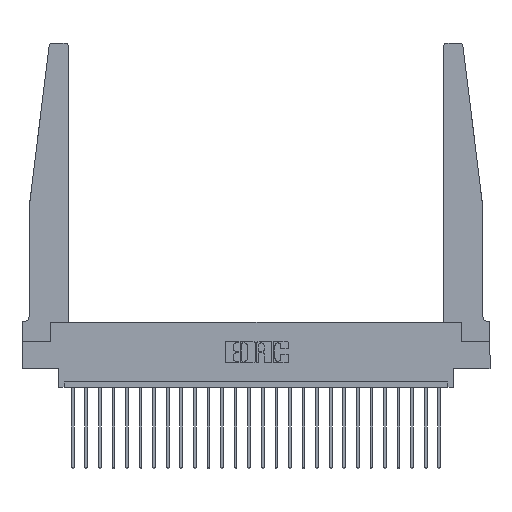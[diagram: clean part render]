
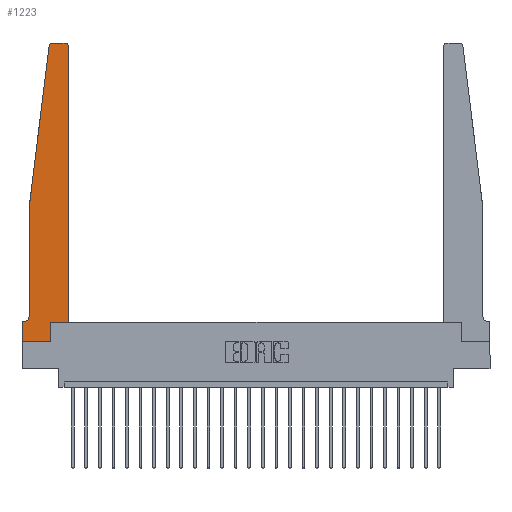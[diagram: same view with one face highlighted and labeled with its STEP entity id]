
A CAD part, top view. The second image highlights one B-rep face of the part: STEP entity #1223.
In plain terms, the highlighted planar face has unit normal (0, 0, 1).
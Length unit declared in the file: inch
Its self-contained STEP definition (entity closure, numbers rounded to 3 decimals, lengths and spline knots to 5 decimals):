
#128 = CARTESIAN_POINT ( 'NONE',  ( 0.425, 0.18, 0.37 ) ) ;
#375 = CIRCLE ( 'NONE', #13480, 0.05 ) ;
#581 = VERTEX_POINT ( 'NONE', #2257 ) ;
#605 = VERTEX_POINT ( 'NONE', #23213 ) ;
#639 = EDGE_CURVE ( 'NONE', #3316, #7666, #14233, .T. ) ;
#1006 = ORIENTED_EDGE ( 'NONE', *, *, #639, .T. ) ;
#1223 = ADVANCED_FACE ( 'NONE', ( #2860 ), #12051, .T. ) ;
#1259 = CARTESIAN_POINT ( 'NONE',  ( 0., 0., 0.37 ) ) ;
#1307 = VERTEX_POINT ( 'NONE', #23726 ) ;
#1462 = ORIENTED_EDGE ( 'NONE', *, *, #21147, .T. ) ;
#1631 = VERTEX_POINT ( 'NONE', #128 ) ;
#1940 = DIRECTION ( 'NONE',  ( 0., 1., 0. ) ) ;
#2257 = CARTESIAN_POINT ( 'NONE',  ( 0.065, 0.2375, 0.37 ) ) ;
#2538 = VERTEX_POINT ( 'NONE', #12047 ) ;
#2718 = VERTEX_POINT ( 'NONE', #4302 ) ;
#2796 = VERTEX_POINT ( 'NONE', #19030 ) ;
#2860 = FACE_OUTER_BOUND ( 'NONE', #19602, .T. ) ;
#3221 = VECTOR ( 'NONE', #15446, 39.37008 ) ;
#3316 = VERTEX_POINT ( 'NONE', #3672 ) ;
#3336 = CARTESIAN_POINT ( 'NONE',  ( 0.065, 0.1875, 0.37 ) ) ;
#3425 = DIRECTION ( 'NONE',  ( -1., 0., 0. ) ) ;
#3672 = CARTESIAN_POINT ( 'NONE',  ( 0., 0.1875, 0.37 ) ) ;
#4198 = VERTEX_POINT ( 'NONE', #4567 ) ;
#4255 = EDGE_CURVE ( 'NONE', #4198, #1307, #8488, .T. ) ;
#4270 = DIRECTION ( 'NONE',  ( 0., 0., 1. ) ) ;
#4302 = CARTESIAN_POINT ( 'NONE',  ( 0.2605, 0., 0.37 ) ) ;
#4433 = LINE ( 'NONE', #18751, #10799 ) ;
#4500 = AXIS2_PLACEMENT_3D ( 'NONE', #13820, #4270, #19492 ) ;
#4567 = CARTESIAN_POINT ( 'NONE',  ( 0.27653, 2.75, 0.37 ) ) ;
#4936 = CARTESIAN_POINT ( 'NONE',  ( 0.015, 0.2375, 0.37 ) ) ;
#5046 = CARTESIAN_POINT ( 'NONE',  ( 0.27653, 2.72, 0.37 ) ) ;
#5383 = EDGE_CURVE ( 'NONE', #2718, #605, #4433, .T. ) ;
#5413 = LINE ( 'NONE', #14546, #8006 ) ;
#5781 = DIRECTION ( 'NONE',  ( 0., 1., 0. ) ) ;
#5889 = DIRECTION ( 'NONE',  ( -0.122, -0.992, 0. ) ) ;
#6013 = CARTESIAN_POINT ( 'NONE',  ( 0.425, 0.18, 0.37 ) ) ;
#6110 = EDGE_CURVE ( 'NONE', #581, #23086, #375, .T. ) ;
#6342 = EDGE_CURVE ( 'NONE', #605, #1631, #12838, .T. ) ;
#6957 = ORIENTED_EDGE ( 'NONE', *, *, #10444, .T. ) ;
#7152 = VECTOR ( 'NONE', #21463, 39.37008 ) ;
#7315 = ORIENTED_EDGE ( 'NONE', *, *, #20209, .T. ) ;
#7651 = LINE ( 'NONE', #3336, #17643 ) ;
#7666 = VERTEX_POINT ( 'NONE', #1259 ) ;
#7957 = AXIS2_PLACEMENT_3D ( 'NONE', #15280, #22581, #18867 ) ;
#8006 = VECTOR ( 'NONE', #3425, 39.37008 ) ;
#8488 = CIRCLE ( 'NONE', #20848, 0.03 ) ;
#9393 = ORIENTED_EDGE ( 'NONE', *, *, #6110, .T. ) ;
#9825 = EDGE_CURVE ( 'NONE', #1631, #2796, #13906, .T. ) ;
#10371 = DIRECTION ( 'NONE',  ( -1., 0., 0. ) ) ;
#10394 = VECTOR ( 'NONE', #15286, 39.37008 ) ;
#10444 = EDGE_CURVE ( 'NONE', #2538, #4198, #5413, .T. ) ;
#10799 = VECTOR ( 'NONE', #1940, 39.37008 ) ;
#11607 = CARTESIAN_POINT ( 'NONE',  ( 0., 0., 0.37 ) ) ;
#11654 = ORIENTED_EDGE ( 'NONE', *, *, #9825, .T. ) ;
#12007 = CIRCLE ( 'NONE', #7957, 0.03 ) ;
#12047 = CARTESIAN_POINT ( 'NONE',  ( 0.395, 2.75, 0.37 ) ) ;
#12051 = PLANE ( 'NONE',  #4500 ) ;
#12712 = VECTOR ( 'NONE', #5889, 39.37008 ) ;
#12769 = ORIENTED_EDGE ( 'NONE', *, *, #16815, .T. ) ;
#12838 = LINE ( 'NONE', #23842, #13147 ) ;
#13147 = VECTOR ( 'NONE', #18865, 39.37008 ) ;
#13480 = AXIS2_PLACEMENT_3D ( 'NONE', #4936, #19993, #10371 ) ;
#13820 = CARTESIAN_POINT ( 'NONE',  ( 0., 0.1875, 0.37 ) ) ;
#13906 = LINE ( 'NONE', #6013, #17472 ) ;
#14233 = LINE ( 'NONE', #11607, #10394 ) ;
#14353 = DIRECTION ( 'NONE',  ( 1., 0., 0. ) ) ;
#14546 = CARTESIAN_POINT ( 'NONE',  ( 0.25, 2.75, 0.37 ) ) ;
#14617 = LINE ( 'NONE', #22761, #3221 ) ;
#15253 = CARTESIAN_POINT ( 'NONE',  ( 0.065, 1.25, 0.37 ) ) ;
#15280 = CARTESIAN_POINT ( 'NONE',  ( 0.395, 2.72, 0.37 ) ) ;
#15286 = DIRECTION ( 'NONE',  ( 0., -1., 0. ) ) ;
#15446 = DIRECTION ( 'NONE',  ( 0., -1., 0. ) ) ;
#16221 = DIRECTION ( 'NONE',  ( 0., 0., 1. ) ) ;
#16271 = CARTESIAN_POINT ( 'NONE',  ( 0.065, 1.25, 0.37 ) ) ;
#16460 = ORIENTED_EDGE ( 'NONE', *, *, #21587, .T. ) ;
#16815 = EDGE_CURVE ( 'NONE', #20340, #581, #14617, .T. ) ;
#17472 = VECTOR ( 'NONE', #5781, 39.37008 ) ;
#17493 = CARTESIAN_POINT ( 'NONE',  ( 0., 0., 0.37 ) ) ;
#17579 = CARTESIAN_POINT ( 'NONE',  ( 0.015, 0.1875, 0.37 ) ) ;
#17643 = VECTOR ( 'NONE', #18329, 39.37008 ) ;
#17776 = LINE ( 'NONE', #15253, #12712 ) ;
#18044 = LINE ( 'NONE', #17493, #7152 ) ;
#18329 = DIRECTION ( 'NONE',  ( -1., 0., 0. ) ) ;
#18715 = ORIENTED_EDGE ( 'NONE', *, *, #5383, .T. ) ;
#18751 = CARTESIAN_POINT ( 'NONE',  ( 0.2605, 0.18, 0.37 ) ) ;
#18865 = DIRECTION ( 'NONE',  ( 1., 0., 0. ) ) ;
#18867 = DIRECTION ( 'NONE',  ( 1., 0., 0. ) ) ;
#19030 = CARTESIAN_POINT ( 'NONE',  ( 0.425, 2.72, 0.37 ) ) ;
#19212 = ORIENTED_EDGE ( 'NONE', *, *, #6342, .T. ) ;
#19298 = ORIENTED_EDGE ( 'NONE', *, *, #21695, .T. ) ;
#19492 = DIRECTION ( 'NONE',  ( 1., 0., 0. ) ) ;
#19602 = EDGE_LOOP ( 'NONE', ( #6957, #22284, #1462, #12769, #9393, #16460, #1006, #7315, #18715, #19212, #11654, #19298 ) ) ;
#19993 = DIRECTION ( 'NONE',  ( 0., 0., -1. ) ) ;
#20209 = EDGE_CURVE ( 'NONE', #7666, #2718, #18044, .T. ) ;
#20340 = VERTEX_POINT ( 'NONE', #16271 ) ;
#20848 = AXIS2_PLACEMENT_3D ( 'NONE', #5046, #16221, #14353 ) ;
#21147 = EDGE_CURVE ( 'NONE', #1307, #20340, #17776, .T. ) ;
#21463 = DIRECTION ( 'NONE',  ( 1., 0., 0. ) ) ;
#21587 = EDGE_CURVE ( 'NONE', #23086, #3316, #7651, .T. ) ;
#21695 = EDGE_CURVE ( 'NONE', #2796, #2538, #12007, .T. ) ;
#22284 = ORIENTED_EDGE ( 'NONE', *, *, #4255, .T. ) ;
#22581 = DIRECTION ( 'NONE',  ( 0., 0., 1. ) ) ;
#22761 = CARTESIAN_POINT ( 'NONE',  ( 0.065, 1.25, 0.37 ) ) ;
#23086 = VERTEX_POINT ( 'NONE', #17579 ) ;
#23213 = CARTESIAN_POINT ( 'NONE',  ( 0.2605, 0.18, 0.37 ) ) ;
#23726 = CARTESIAN_POINT ( 'NONE',  ( 0.24675, 2.72367, 0.37 ) ) ;
#23842 = CARTESIAN_POINT ( 'NONE',  ( 0.425, 0.18, 0.37 ) ) ;
